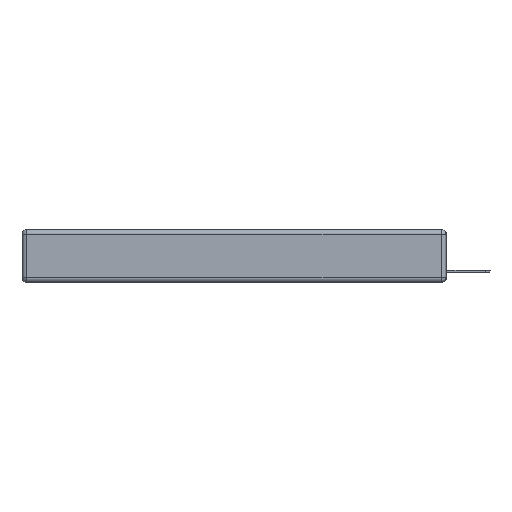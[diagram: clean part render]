
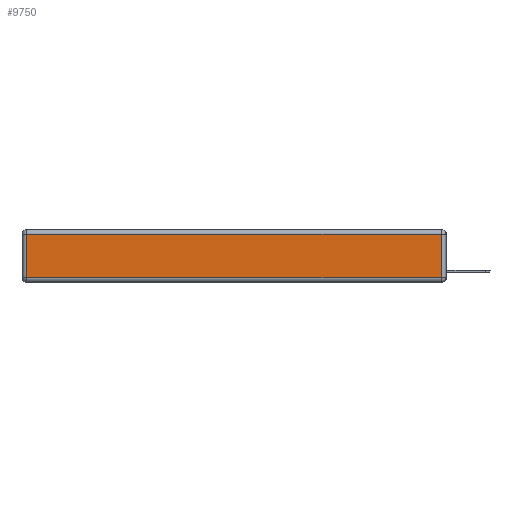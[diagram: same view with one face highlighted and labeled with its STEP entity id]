
A CAD part, left-side view. The second image highlights one B-rep face of the part: STEP entity #9750.
In plain terms, the highlighted planar face has unit normal (-1, 0, 0).
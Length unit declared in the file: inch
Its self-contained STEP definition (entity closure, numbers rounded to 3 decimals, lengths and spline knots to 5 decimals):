
#212 = ORIENTED_EDGE ( 'NONE', *, *, #12505, .T. ) ;
#626 = VERTEX_POINT ( 'NONE', #9381 ) ;
#1208 = ORIENTED_EDGE ( 'NONE', *, *, #9933, .T. ) ;
#2226 = CARTESIAN_POINT ( 'NONE',  ( 0., 0.03, -0.03 ) ) ;
#2410 = DIRECTION ( 'NONE',  ( 0., 0., 1. ) ) ;
#3239 = LINE ( 'NONE', #5144, #12531 ) ;
#3290 = ORIENTED_EDGE ( 'NONE', *, *, #3805, .T. ) ;
#3363 = DIRECTION ( 'NONE',  ( 0., -1., 0. ) ) ;
#3805 = EDGE_CURVE ( 'NONE', #6427, #11446, #8977, .T. ) ;
#4025 = VECTOR ( 'NONE', #8586, 39.37008 ) ;
#4788 = CARTESIAN_POINT ( 'NONE',  ( 0., 2.75, -0.03 ) ) ;
#5144 = CARTESIAN_POINT ( 'NONE',  ( 0., 0., -0.313 ) ) ;
#5376 = ORIENTED_EDGE ( 'NONE', *, *, #12376, .T. ) ;
#5929 = LINE ( 'NONE', #12572, #4025 ) ;
#6011 = CARTESIAN_POINT ( 'NONE',  ( 0., 2.72, -0.313 ) ) ;
#6139 = LINE ( 'NONE', #4788, #10076 ) ;
#6427 = VERTEX_POINT ( 'NONE', #9113 ) ;
#6492 = PLANE ( 'NONE',  #7753 ) ;
#7318 = DIRECTION ( 'NONE',  ( 0., 0., -1. ) ) ;
#7415 = FACE_OUTER_BOUND ( 'NONE', #12235, .T. ) ;
#7753 = AXIS2_PLACEMENT_3D ( 'NONE', #8392, #8484, #2410 ) ;
#8392 = CARTESIAN_POINT ( 'NONE',  ( 0., 0., -0.343 ) ) ;
#8484 = DIRECTION ( 'NONE',  ( -1., 0., 0. ) ) ;
#8586 = DIRECTION ( 'NONE',  ( 0., 0., 1. ) ) ;
#8912 = DIRECTION ( 'NONE',  ( 0., 1., 0. ) ) ;
#8977 = LINE ( 'NONE', #9308, #11465 ) ;
#9113 = CARTESIAN_POINT ( 'NONE',  ( 0., 2.72, -0.03 ) ) ;
#9308 = CARTESIAN_POINT ( 'NONE',  ( 0., 2.72, -0.343 ) ) ;
#9381 = CARTESIAN_POINT ( 'NONE',  ( 0., 0.03, -0.313 ) ) ;
#9750 = ADVANCED_FACE ( 'NONE', ( #7415 ), #6492, .T. ) ;
#9933 = EDGE_CURVE ( 'NONE', #11773, #6427, #6139, .T. ) ;
#10076 = VECTOR ( 'NONE', #8912, 39.37008 ) ;
#11446 = VERTEX_POINT ( 'NONE', #6011 ) ;
#11465 = VECTOR ( 'NONE', #7318, 39.37008 ) ;
#11773 = VERTEX_POINT ( 'NONE', #2226 ) ;
#12235 = EDGE_LOOP ( 'NONE', ( #5376, #212, #1208, #3290 ) ) ;
#12376 = EDGE_CURVE ( 'NONE', #11446, #626, #3239, .T. ) ;
#12505 = EDGE_CURVE ( 'NONE', #626, #11773, #5929, .T. ) ;
#12531 = VECTOR ( 'NONE', #3363, 39.37008 ) ;
#12572 = CARTESIAN_POINT ( 'NONE',  ( 0., 0.03, -0.343 ) ) ;
